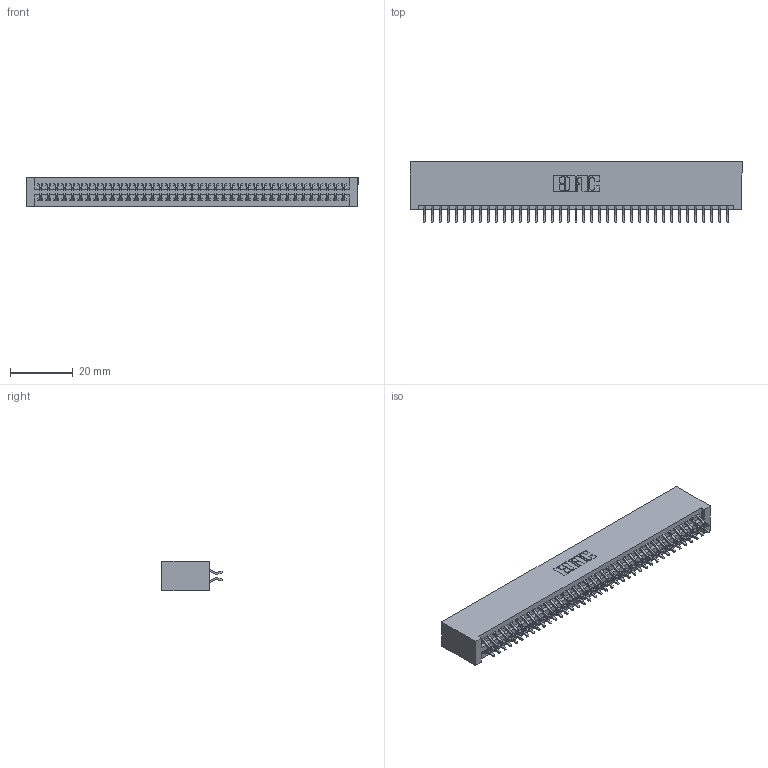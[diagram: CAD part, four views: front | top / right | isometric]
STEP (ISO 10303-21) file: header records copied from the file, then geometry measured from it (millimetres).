
FILE_DESCRIPTION (( 'STEP AP203' ), '1' );
FILE_NAME ('395-078-556-201.STEP', '2019-10-25T02:58:52', ( '' ), ( '' ), 'SwSTEP 2.0', 'SolidWorks 2016', '' );
FILE_SCHEMA (( 'CONFIG_CONTROL_DESIGN' ));
Length unit declared in the file: inch
Products named in the file (3): 345-292-001_556 Tail; 395-078-556-201; 345 Part_No Mounting Lugs
Assembly tree (79 placements, depth 2):
  395-078-556-201
    345 Part_No Mounting Lugs
    345-292-001_556 Tail  x78
Bounding box: 105.66 x 19.24 x 9.4 mm (x, y, z)
Volume: 10849.3 mm3; surface area: 16213.9 mm2
Topology: 79 solids, 79 shells, 4486 faces, 13343 edges, 8790 vertices
Faces by surface type: plane 2962, cylinder 1524
Entity records: 30947 total; most frequent: CARTESIAN_POINT 5204, ORIENTED_EDGE 5126, DIRECTION 4575, EDGE_CURVE 2563, LINE 2275, VECTOR 2275, VERTEX_POINT 1706, AXIS2_PLACEMENT_3D 1150
